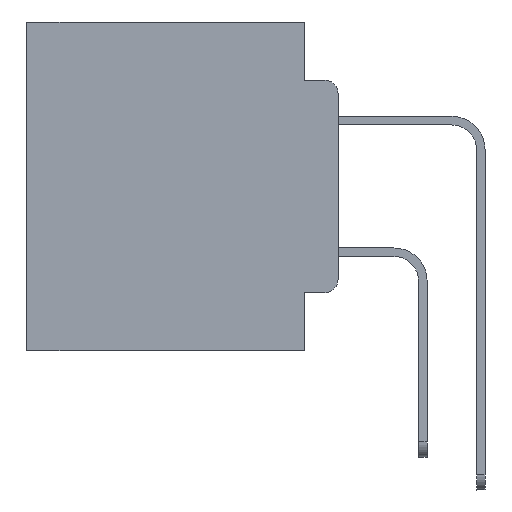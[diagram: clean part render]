
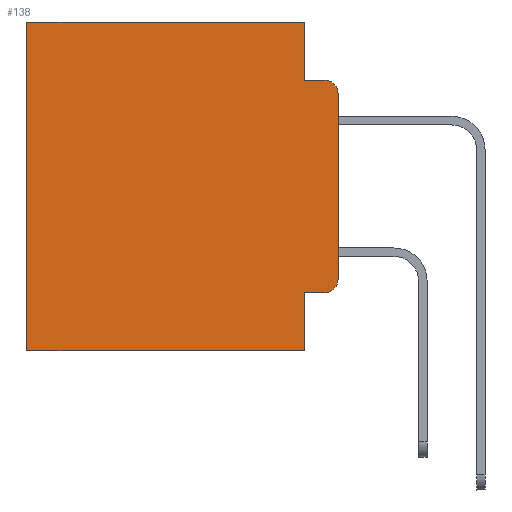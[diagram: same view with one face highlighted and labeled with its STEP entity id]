
A CAD part, left-side view. The second image highlights one B-rep face of the part: STEP entity #138.
In plain terms, the highlighted planar face has unit normal (-1, 0, 0).
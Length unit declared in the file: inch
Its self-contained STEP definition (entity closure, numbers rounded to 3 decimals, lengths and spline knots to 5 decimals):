
#138 = ADVANCED_FACE ( 'NONE', ( #12352 ), #21886, .F. ) ;
#139 = EDGE_CURVE ( 'NONE', #19998, #26500, #7651, .T. ) ;
#401 = CIRCLE ( 'NONE', #3888, 0.02 ) ;
#436 = CARTESIAN_POINT ( 'NONE',  ( 0.298, 0., 0. ) ) ;
#636 = VERTEX_POINT ( 'NONE', #24339 ) ;
#1396 = CARTESIAN_POINT ( 'NONE',  ( 0.298, 0., -0.5 ) ) ;
#1496 = DIRECTION ( 'NONE',  ( 0., 0., -1. ) ) ;
#3848 = ORIENTED_EDGE ( 'NONE', *, *, #25139, .T. ) ;
#3888 = AXIS2_PLACEMENT_3D ( 'NONE', #5166, #9868, #24397 ) ;
#4171 = LINE ( 'NONE', #23401, #27961 ) ;
#4867 = VERTEX_POINT ( 'NONE', #22192 ) ;
#5166 = CARTESIAN_POINT ( 'NONE',  ( 0.298, 0.02, -0.1085 ) ) ;
#5304 = DIRECTION ( 'NONE',  ( 0., 0., -1. ) ) ;
#6071 = LINE ( 'NONE', #11066, #23528 ) ;
#6621 = CIRCLE ( 'NONE', #25106, 0.02 ) ;
#6679 = DIRECTION ( 'NONE',  ( 0., 1., 0. ) ) ;
#6729 = DIRECTION ( 'NONE',  ( 0., 1., 0. ) ) ;
#7369 = ORIENTED_EDGE ( 'NONE', *, *, #8246, .F. ) ;
#7651 = LINE ( 'NONE', #17180, #24017 ) ;
#8053 = AXIS2_PLACEMENT_3D ( 'NONE', #436, #9997, #29033 ) ;
#8246 = EDGE_CURVE ( 'NONE', #24102, #636, #15309, .T. ) ;
#9160 = EDGE_CURVE ( 'NONE', #22749, #18671, #29694, .T. ) ;
#9401 = VERTEX_POINT ( 'NONE', #11567 ) ;
#9868 = DIRECTION ( 'NONE',  ( -1., 0., 0. ) ) ;
#9997 = DIRECTION ( 'NONE',  ( 1., 0., 0. ) ) ;
#10041 = ORIENTED_EDGE ( 'NONE', *, *, #29757, .F. ) ;
#10198 = DIRECTION ( 'NONE',  ( 0., 0., -1. ) ) ;
#10259 = CARTESIAN_POINT ( 'NONE',  ( 0.298, 0.051, -0.0885 ) ) ;
#10914 = DIRECTION ( 'NONE',  ( 0., 0., -1. ) ) ;
#11066 = CARTESIAN_POINT ( 'NONE',  ( 0.298, 0.051, 0. ) ) ;
#11456 = CARTESIAN_POINT ( 'NONE',  ( 0.298, 0.473, -0.5 ) ) ;
#11567 = CARTESIAN_POINT ( 'NONE',  ( 0.298, 0.02, -0.4115 ) ) ;
#11855 = ORIENTED_EDGE ( 'NONE', *, *, #9160, .F. ) ;
#12018 = EDGE_CURVE ( 'NONE', #22749, #9401, #12260, .T. ) ;
#12260 = LINE ( 'NONE', #22254, #27834 ) ;
#12352 = FACE_OUTER_BOUND ( 'NONE', #24550, .T. ) ;
#12724 = DIRECTION ( 'NONE',  ( 0., -1., 0. ) ) ;
#13422 = CARTESIAN_POINT ( 'NONE',  ( 0.298, 0.473, 0. ) ) ;
#13730 = LINE ( 'NONE', #16210, #20504 ) ;
#14272 = VECTOR ( 'NONE', #10198, 39.37008 ) ;
#14848 = EDGE_CURVE ( 'NONE', #4867, #20112, #13730, .T. ) ;
#14882 = EDGE_CURVE ( 'NONE', #20112, #19383, #4171, .T. ) ;
#14891 = DIRECTION ( 'NONE',  ( 0., 0., -1. ) ) ;
#15115 = VECTOR ( 'NONE', #6729, 39.37008 ) ;
#15309 = LINE ( 'NONE', #24683, #28757 ) ;
#16210 = CARTESIAN_POINT ( 'NONE',  ( 0.298, 0., 0. ) ) ;
#16710 = CARTESIAN_POINT ( 'NONE',  ( 0.298, 0.051, -0.5 ) ) ;
#16735 = ORIENTED_EDGE ( 'NONE', *, *, #14882, .T. ) ;
#17180 = CARTESIAN_POINT ( 'NONE',  ( 0.298, 0., 0. ) ) ;
#18248 = EDGE_CURVE ( 'NONE', #9401, #26500, #6621, .T. ) ;
#18671 = VERTEX_POINT ( 'NONE', #16710 ) ;
#18690 = ORIENTED_EDGE ( 'NONE', *, *, #30594, .F. ) ;
#19273 = CARTESIAN_POINT ( 'NONE',  ( 0.298, 0., -0.3915 ) ) ;
#19383 = VERTEX_POINT ( 'NONE', #11456 ) ;
#19981 = DIRECTION ( 'NONE',  ( 0., -1., 0. ) ) ;
#19998 = VERTEX_POINT ( 'NONE', #22497 ) ;
#20112 = VERTEX_POINT ( 'NONE', #13422 ) ;
#20504 = VECTOR ( 'NONE', #6679, 39.37008 ) ;
#21444 = ORIENTED_EDGE ( 'NONE', *, *, #14848, .T. ) ;
#21886 = PLANE ( 'NONE',  #8053 ) ;
#21933 = DIRECTION ( 'NONE',  ( -1., 0., 0. ) ) ;
#22192 = CARTESIAN_POINT ( 'NONE',  ( 0.298, 0.051, 0. ) ) ;
#22254 = CARTESIAN_POINT ( 'NONE',  ( 0.298, 0.051, -0.4115 ) ) ;
#22497 = CARTESIAN_POINT ( 'NONE',  ( 0.298, 0., -0.1085 ) ) ;
#22543 = CARTESIAN_POINT ( 'NONE',  ( 0.298, 0.051, -0.4115 ) ) ;
#22749 = VERTEX_POINT ( 'NONE', #22543 ) ;
#22835 = CARTESIAN_POINT ( 'NONE',  ( 0.298, 0.051, 0. ) ) ;
#22837 = LINE ( 'NONE', #1396, #15115 ) ;
#23269 = ORIENTED_EDGE ( 'NONE', *, *, #18248, .T. ) ;
#23401 = CARTESIAN_POINT ( 'NONE',  ( 0.298, 0.473, 0. ) ) ;
#23528 = VECTOR ( 'NONE', #10914, 39.37008 ) ;
#24017 = VECTOR ( 'NONE', #5304, 39.37008 ) ;
#24102 = VERTEX_POINT ( 'NONE', #10259 ) ;
#24339 = CARTESIAN_POINT ( 'NONE',  ( 0.298, 0.02, -0.0885 ) ) ;
#24397 = DIRECTION ( 'NONE',  ( 0., 0., -1. ) ) ;
#24550 = EDGE_LOOP ( 'NONE', ( #29616, #3848, #7369, #10041, #21444, #16735, #18690, #11855, #30583, #23269 ) ) ;
#24683 = CARTESIAN_POINT ( 'NONE',  ( 0.298, 0.051, -0.0885 ) ) ;
#25106 = AXIS2_PLACEMENT_3D ( 'NONE', #26283, #21933, #14891 ) ;
#25139 = EDGE_CURVE ( 'NONE', #19998, #636, #401, .T. ) ;
#26283 = CARTESIAN_POINT ( 'NONE',  ( 0.298, 0.02, -0.3915 ) ) ;
#26500 = VERTEX_POINT ( 'NONE', #19273 ) ;
#27834 = VECTOR ( 'NONE', #12724, 39.37008 ) ;
#27961 = VECTOR ( 'NONE', #1496, 39.37008 ) ;
#28757 = VECTOR ( 'NONE', #19981, 39.37008 ) ;
#29033 = DIRECTION ( 'NONE',  ( 0., 0., -1. ) ) ;
#29616 = ORIENTED_EDGE ( 'NONE', *, *, #139, .F. ) ;
#29694 = LINE ( 'NONE', #22835, #14272 ) ;
#29757 = EDGE_CURVE ( 'NONE', #4867, #24102, #6071, .T. ) ;
#30583 = ORIENTED_EDGE ( 'NONE', *, *, #12018, .T. ) ;
#30594 = EDGE_CURVE ( 'NONE', #18671, #19383, #22837, .T. ) ;
